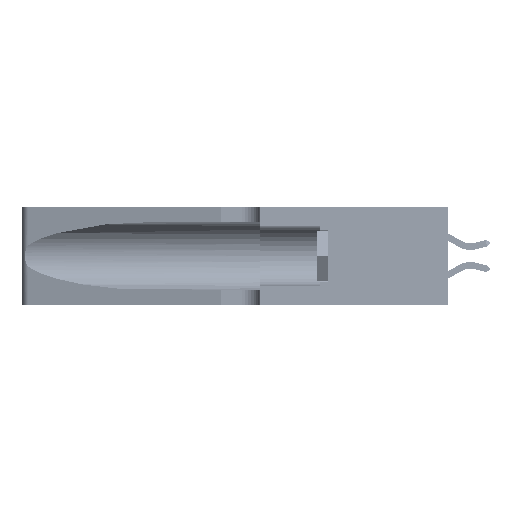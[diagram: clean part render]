
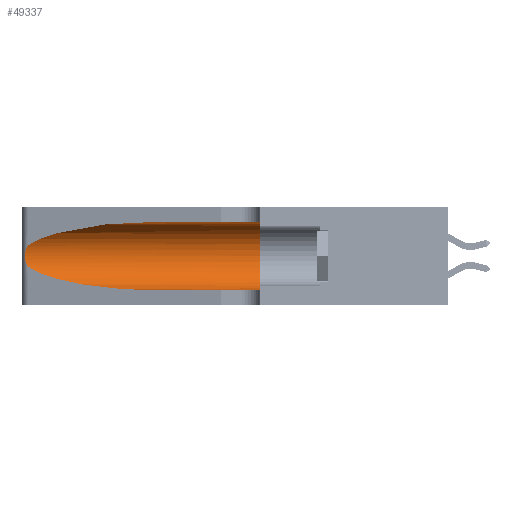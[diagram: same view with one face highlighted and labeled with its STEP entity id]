
A CAD part, left-side view. The second image highlights one B-rep face of the part: STEP entity #49337.
In plain terms, the highlighted cylindrical face has radius 3.308 mm (diameter 6.617 mm), a partial arc.
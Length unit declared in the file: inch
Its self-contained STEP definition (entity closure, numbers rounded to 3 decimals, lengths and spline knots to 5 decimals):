
#749 = CARTESIAN_POINT ( 'NONE',  ( 0.1305, 0.72297, 0.31525 ) ) ;
#1052 = EDGE_CURVE ( 'NONE', #45369, #25799, #24336, .T. ) ;
#4263 = CARTESIAN_POINT ( 'NONE',  ( 0.1305, 0.72297, 0.05475 ) ) ;
#5763 = VERTEX_POINT ( 'NONE', #38471 ) ;
#6614 = CARTESIAN_POINT ( 'NONE',  ( 0.25854, 1.2359, 0.20912 ) ) ;
#6800 = CARTESIAN_POINT ( 'NONE',  ( 0.26018, 1.23835, 0.19895 ) ) ;
#6981 = CARTESIAN_POINT ( 'NONE',  ( 0.25555, 1.22993, 0.14849 ) ) ;
#7669 = B_SPLINE_CURVE_WITH_KNOTS ( 'NONE', 3,
 ( #44821, #32155, #44434, #31793, #6614, #6800, #36272, #10873, #50041, #20137, #49850, #49662, #6981, #24405 ),
 .UNSPECIFIED., .F., .F.,
 ( 4, 2, 2, 2, 2, 2, 4 ),
 ( 0., 0.00027, 0.00053, 0.00107, 0.0016, 0.00187, 0.00214 ),
 .UNSPECIFIED. ) ;
#8235 = VERTEX_POINT ( 'NONE', #24404 ) ;
#10873 = CARTESIAN_POINT ( 'NONE',  ( 0.26075, 1.23896, 0.178 ) ) ;
#11228 = DIRECTION ( 'NONE',  ( 0., 0., -1. ) ) ;
#12678 = CARTESIAN_POINT ( 'NONE',  ( 0.1305, 1.61858, 0.05475 ) ) ;
#16420 = ORIENTED_EDGE ( 'NONE', *, *, #34099, .F. ) ;
#17057 = ORIENTED_EDGE ( 'NONE', *, *, #51814, .F. ) ;
#17095 = VECTOR ( 'NONE', #42548, 39.37008 ) ;
#18928 = AXIS2_PLACEMENT_3D ( 'NONE', #45176, #28840, #11228 ) ;
#20137 = CARTESIAN_POINT ( 'NONE',  ( 0.25856, 1.23593, 0.16098 ) ) ;
#21238 = CYLINDRICAL_SURFACE ( 'NONE', #18928, 0.13025 ) ;
#22057 = EDGE_CURVE ( 'NONE', #5763, #45369, #7669, .T. ) ;
#22071 = VECTOR ( 'NONE', #47202, 39.37008 ) ;
#23790 = CARTESIAN_POINT ( 'NONE',  ( 0.25487, 1.22718, 0.14631 ) ) ;
#24336 =( BOUNDED_CURVE ( )  B_SPLINE_CURVE ( 3, ( #46568, #50879, #29637, #4263 ),
 .UNSPECIFIED., .F., .F. ) 
 B_SPLINE_CURVE_WITH_KNOTS ( ( 4, 4 ),
 ( 3.44316, 4.71239 ),
 .UNSPECIFIED. ) 
 CURVE ( )  GEOMETRIC_REPRESENTATION_ITEM ( )  RATIONAL_B_SPLINE_CURVE ( ( 1., 0.87, 0.87, 1. ) ) 
 REPRESENTATION_ITEM ( '' )  );
#24387 = EDGE_CURVE ( 'NONE', #25799, #8235, #26689, .T. ) ;
#24404 = CARTESIAN_POINT ( 'NONE',  ( 0.1305, 0.35, 0.05475 ) ) ;
#24405 = CARTESIAN_POINT ( 'NONE',  ( 0.25487, 1.22718, 0.14631 ) ) ;
#24826 = ORIENTED_EDGE ( 'NONE', *, *, #22057, .T. ) ;
#25363 = CARTESIAN_POINT ( 'NONE',  ( 0.1305, 0.72297, 0.31525 ) ) ;
#25799 = VERTEX_POINT ( 'NONE', #32959 ) ;
#26689 = LINE ( 'NONE', #12678, #22071 ) ;
#27558 = CIRCLE ( 'NONE', #44928, 0.13025 ) ;
#27810 = ORIENTED_EDGE ( 'NONE', *, *, #1052, .T. ) ;
#28840 = DIRECTION ( 'NONE',  ( 0., -1., 0. ) ) ;
#29637 = CARTESIAN_POINT ( 'NONE',  ( 0.18966, 0.96281, 0.05475 ) ) ;
#31352 = EDGE_CURVE ( 'NONE', #52375, #5763, #33122, .T. ) ;
#31793 = CARTESIAN_POINT ( 'NONE',  ( 0.25787, 1.23484, 0.2124 ) ) ;
#32155 = CARTESIAN_POINT ( 'NONE',  ( 0.25555, 1.22994, 0.2215 ) ) ;
#32782 = DIRECTION ( 'NONE',  ( 0., 1., 0. ) ) ;
#32848 = VERTEX_POINT ( 'NONE', #38199 ) ;
#32959 = CARTESIAN_POINT ( 'NONE',  ( 0.1305, 0.72297, 0.05475 ) ) ;
#33122 =( BOUNDED_CURVE ( )  B_SPLINE_CURVE ( 3, ( #25363, #50263, #33660, #46338 ),
 .UNSPECIFIED., .F., .F. ) 
 B_SPLINE_CURVE_WITH_KNOTS ( ( 4, 4 ),
 ( 1.5708, 2.84003 ),
 .UNSPECIFIED. ) 
 CURVE ( )  GEOMETRIC_REPRESENTATION_ITEM ( )  RATIONAL_B_SPLINE_CURVE ( ( 1., 0.87, 0.87, 1. ) ) 
 REPRESENTATION_ITEM ( '' )  );
#33154 = FACE_OUTER_BOUND ( 'NONE', #42499, .T. ) ;
#33602 = CARTESIAN_POINT ( 'NONE',  ( 0.1305, 1.61858, 0.31525 ) ) ;
#33660 = CARTESIAN_POINT ( 'NONE',  ( 0.2373, 1.15595, 0.28018 ) ) ;
#34099 = EDGE_CURVE ( 'NONE', #52375, #32848, #52352, .T. ) ;
#34359 = CARTESIAN_POINT ( 'NONE',  ( 0.1305, 0.35, 0.185 ) ) ;
#36272 = CARTESIAN_POINT ( 'NONE',  ( 0.26075, 1.23896, 0.19203 ) ) ;
#36876 = ORIENTED_EDGE ( 'NONE', *, *, #31352, .T. ) ;
#38199 = CARTESIAN_POINT ( 'NONE',  ( 0.1305, 0.35, 0.31525 ) ) ;
#38471 = CARTESIAN_POINT ( 'NONE',  ( 0.25487, 1.22718, 0.22369 ) ) ;
#38618 = ORIENTED_EDGE ( 'NONE', *, *, #24387, .T. ) ;
#42027 = DIRECTION ( 'NONE',  ( 0., 0., 1. ) ) ;
#42499 = EDGE_LOOP ( 'NONE', ( #36876, #24826, #27810, #38618, #17057, #16420 ) ) ;
#42548 = DIRECTION ( 'NONE',  ( 0., -1., 0. ) ) ;
#44434 = CARTESIAN_POINT ( 'NONE',  ( 0.25639, 1.23184, 0.21858 ) ) ;
#44821 = CARTESIAN_POINT ( 'NONE',  ( 0.25487, 1.22718, 0.22369 ) ) ;
#44928 = AXIS2_PLACEMENT_3D ( 'NONE', #34359, #32782, #42027 ) ;
#45176 = CARTESIAN_POINT ( 'NONE',  ( 0.1305, 1.61858, 0.185 ) ) ;
#45369 = VERTEX_POINT ( 'NONE', #23790 ) ;
#46338 = CARTESIAN_POINT ( 'NONE',  ( 0.25487, 1.22718, 0.22369 ) ) ;
#46568 = CARTESIAN_POINT ( 'NONE',  ( 0.25487, 1.22718, 0.14631 ) ) ;
#47202 = DIRECTION ( 'NONE',  ( 0., -1., 0. ) ) ;
#49337 = ADVANCED_FACE ( 'NONE', ( #33154 ), #21238, .F. ) ;
#49662 = CARTESIAN_POINT ( 'NONE',  ( 0.25639, 1.23186, 0.15144 ) ) ;
#49850 = CARTESIAN_POINT ( 'NONE',  ( 0.25789, 1.23486, 0.15765 ) ) ;
#50041 = CARTESIAN_POINT ( 'NONE',  ( 0.26017, 1.23833, 0.17102 ) ) ;
#50263 = CARTESIAN_POINT ( 'NONE',  ( 0.18966, 0.96281, 0.31525 ) ) ;
#50879 = CARTESIAN_POINT ( 'NONE',  ( 0.2373, 1.15595, 0.08982 ) ) ;
#51814 = EDGE_CURVE ( 'NONE', #32848, #8235, #27558, .T. ) ;
#52352 = LINE ( 'NONE', #33602, #17095 ) ;
#52375 = VERTEX_POINT ( 'NONE', #749 ) ;
